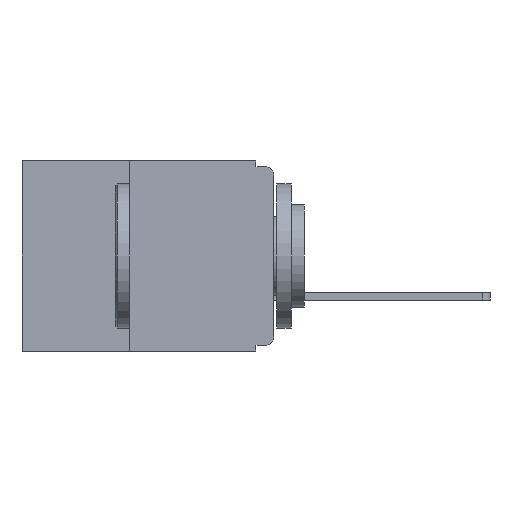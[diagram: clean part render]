
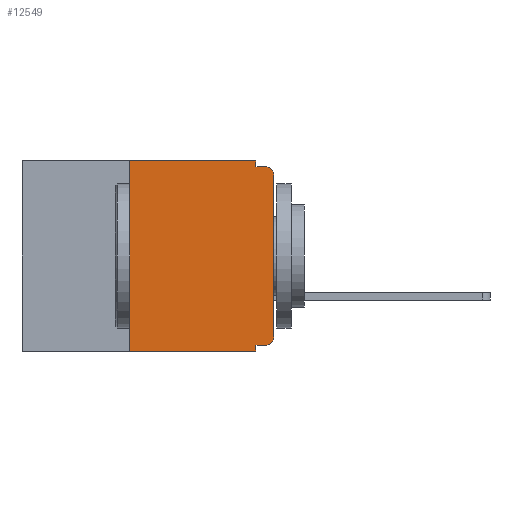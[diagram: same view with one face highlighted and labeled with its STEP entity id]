
A CAD part, left-side view. The second image highlights one B-rep face of the part: STEP entity #12549.
In plain terms, the highlighted planar face has unit normal (-1, 0, 0).
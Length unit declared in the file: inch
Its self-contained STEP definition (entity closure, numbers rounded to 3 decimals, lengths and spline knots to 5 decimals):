
#101 = CARTESIAN_POINT ( 'NONE',  ( 0., 0.015, -0.01 ) ) ;
#760 = VERTEX_POINT ( 'NONE', #7126 ) ;
#884 = ORIENTED_EDGE ( 'NONE', *, *, #8623, .T. ) ;
#936 = CARTESIAN_POINT ( 'NONE',  ( 0., 0.015, -0.025 ) ) ;
#975 = VERTEX_POINT ( 'NONE', #8055 ) ;
#1102 = ORIENTED_EDGE ( 'NONE', *, *, #3043, .T. ) ;
#1153 = DIRECTION ( 'NONE',  ( 0., 0., 1. ) ) ;
#1825 = VECTOR ( 'NONE', #2059, 39.37008 ) ;
#1835 = ORIENTED_EDGE ( 'NONE', *, *, #17041, .F. ) ;
#2059 = DIRECTION ( 'NONE',  ( 0., -1., 0. ) ) ;
#2076 = VECTOR ( 'NONE', #13876, 39.37008 ) ;
#2457 = VECTOR ( 'NONE', #7028, 39.37008 ) ;
#2703 = EDGE_CURVE ( 'NONE', #8358, #17464, #20659, .T. ) ;
#3043 = EDGE_CURVE ( 'NONE', #24899, #8358, #11768, .T. ) ;
#3267 = DIRECTION ( 'NONE',  ( 0., 0., -1. ) ) ;
#4340 = ORIENTED_EDGE ( 'NONE', *, *, #13823, .F. ) ;
#5525 = VECTOR ( 'NONE', #1153, 39.37008 ) ;
#6456 = DIRECTION ( 'NONE',  ( 0., -1., 0. ) ) ;
#6626 = CARTESIAN_POINT ( 'NONE',  ( 0., 0., 0. ) ) ;
#7028 = DIRECTION ( 'NONE',  ( 0., 0., 1. ) ) ;
#7126 = CARTESIAN_POINT ( 'NONE',  ( 0., 0.25, -0.33 ) ) ;
#7574 = CARTESIAN_POINT ( 'NONE',  ( 0., 0.25, 0. ) ) ;
#7932 = LINE ( 'NONE', #15703, #1825 ) ;
#8055 = CARTESIAN_POINT ( 'NONE',  ( 0., 0.031, -0.33 ) ) ;
#8171 = LINE ( 'NONE', #20662, #2076 ) ;
#8358 = VERTEX_POINT ( 'NONE', #19328 ) ;
#8623 = EDGE_CURVE ( 'NONE', #760, #975, #7932, .T. ) ;
#8803 = ORIENTED_EDGE ( 'NONE', *, *, #26982, .F. ) ;
#9528 = CARTESIAN_POINT ( 'NONE',  ( 0., 0.031, -0.01 ) ) ;
#10183 = LINE ( 'NONE', #15673, #20881 ) ;
#10426 = EDGE_CURVE ( 'NONE', #17464, #25818, #22307, .T. ) ;
#10459 = EDGE_CURVE ( 'NONE', #28542, #18114, #26963, .T. ) ;
#10460 = CARTESIAN_POINT ( 'NONE',  ( 0., 0.015, -0.32 ) ) ;
#10686 = VECTOR ( 'NONE', #6456, 39.37008 ) ;
#11396 = ORIENTED_EDGE ( 'NONE', *, *, #10459, .F. ) ;
#11759 = CARTESIAN_POINT ( 'NONE',  ( 0., 0.437, 0. ) ) ;
#11768 = CIRCLE ( 'NONE', #18294, 0.015 ) ;
#11879 = CARTESIAN_POINT ( 'NONE',  ( 0., 0.031, -0.33 ) ) ;
#12506 = DIRECTION ( 'NONE',  ( 0., 0., -1. ) ) ;
#12549 = ADVANCED_FACE ( 'NONE', ( #28264 ), #23153, .F. ) ;
#12774 = VECTOR ( 'NONE', #25604, 39.37008 ) ;
#12856 = VERTEX_POINT ( 'NONE', #21859 ) ;
#12965 = EDGE_CURVE ( 'NONE', #18114, #25818, #28235, .T. ) ;
#13719 = CARTESIAN_POINT ( 'NONE',  ( 0., 0.031, 0. ) ) ;
#13740 = EDGE_CURVE ( 'NONE', #20102, #28542, #8171, .T. ) ;
#13823 = EDGE_CURVE ( 'NONE', #12856, #975, #23520, .T. ) ;
#13876 = DIRECTION ( 'NONE',  ( 0., -1., 0. ) ) ;
#14039 = DIRECTION ( 'NONE',  ( 0., 0., -1. ) ) ;
#15673 = CARTESIAN_POINT ( 'NONE',  ( 0., 0., -0.32 ) ) ;
#15703 = CARTESIAN_POINT ( 'NONE',  ( 0., 0.437, -0.33 ) ) ;
#16879 = DIRECTION ( 'NONE',  ( -1., 0., 0. ) ) ;
#17041 = EDGE_CURVE ( 'NONE', #24899, #12856, #10183, .T. ) ;
#17464 = VERTEX_POINT ( 'NONE', #24005 ) ;
#17950 = DIRECTION ( 'NONE',  ( 0., 1., 0. ) ) ;
#18114 = VERTEX_POINT ( 'NONE', #9528 ) ;
#18294 = AXIS2_PLACEMENT_3D ( 'NONE', #21054, #21331, #21323 ) ;
#18575 = AXIS2_PLACEMENT_3D ( 'NONE', #936, #16879, #3267 ) ;
#18882 = EDGE_LOOP ( 'NONE', ( #27697, #29016, #19391, #11396, #20592, #8803, #884, #4340, #1835, #1102 ) ) ;
#19328 = CARTESIAN_POINT ( 'NONE',  ( 0., 0., -0.305 ) ) ;
#19391 = ORIENTED_EDGE ( 'NONE', *, *, #12965, .F. ) ;
#20095 = CARTESIAN_POINT ( 'NONE',  ( 0., 0., -0.01 ) ) ;
#20102 = VERTEX_POINT ( 'NONE', #7574 ) ;
#20592 = ORIENTED_EDGE ( 'NONE', *, *, #13740, .F. ) ;
#20659 = LINE ( 'NONE', #6626, #2457 ) ;
#20662 = CARTESIAN_POINT ( 'NONE',  ( 0., 0.437, 0. ) ) ;
#20755 = AXIS2_PLACEMENT_3D ( 'NONE', #11759, #27766, #14039 ) ;
#20881 = VECTOR ( 'NONE', #17950, 39.37008 ) ;
#21054 = CARTESIAN_POINT ( 'NONE',  ( 0., 0.015, -0.305 ) ) ;
#21323 = DIRECTION ( 'NONE',  ( 0., 0., -1. ) ) ;
#21331 = DIRECTION ( 'NONE',  ( -1., 0., 0. ) ) ;
#21598 = VECTOR ( 'NONE', #12506, 39.37008 ) ;
#21859 = CARTESIAN_POINT ( 'NONE',  ( 0., 0.031, -0.32 ) ) ;
#22307 = CIRCLE ( 'NONE', #18575, 0.015 ) ;
#23153 = PLANE ( 'NONE',  #20755 ) ;
#23520 = LINE ( 'NONE', #11879, #12774 ) ;
#23763 = LINE ( 'NONE', #26262, #5525 ) ;
#24005 = CARTESIAN_POINT ( 'NONE',  ( 0., 0., -0.025 ) ) ;
#24899 = VERTEX_POINT ( 'NONE', #10460 ) ;
#25604 = DIRECTION ( 'NONE',  ( 0., 0., -1. ) ) ;
#25818 = VERTEX_POINT ( 'NONE', #101 ) ;
#26254 = CARTESIAN_POINT ( 'NONE',  ( 0., 0.031, 0. ) ) ;
#26262 = CARTESIAN_POINT ( 'NONE',  ( 0., 0.25, -0.33 ) ) ;
#26963 = LINE ( 'NONE', #26254, #21598 ) ;
#26982 = EDGE_CURVE ( 'NONE', #760, #20102, #23763, .T. ) ;
#27697 = ORIENTED_EDGE ( 'NONE', *, *, #2703, .T. ) ;
#27766 = DIRECTION ( 'NONE',  ( 1., 0., 0. ) ) ;
#28235 = LINE ( 'NONE', #20095, #10686 ) ;
#28264 = FACE_OUTER_BOUND ( 'NONE', #18882, .T. ) ;
#28542 = VERTEX_POINT ( 'NONE', #13719 ) ;
#29016 = ORIENTED_EDGE ( 'NONE', *, *, #10426, .T. ) ;
